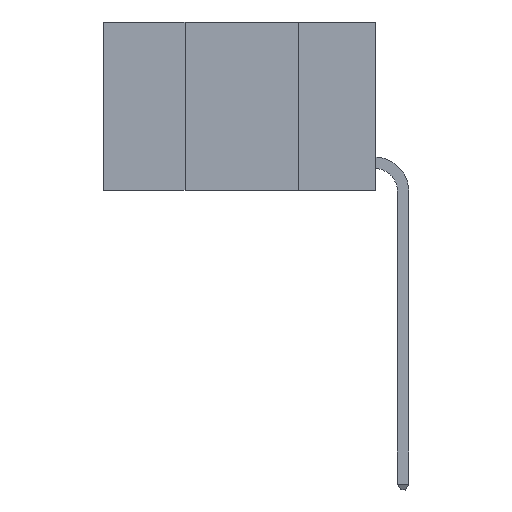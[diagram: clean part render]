
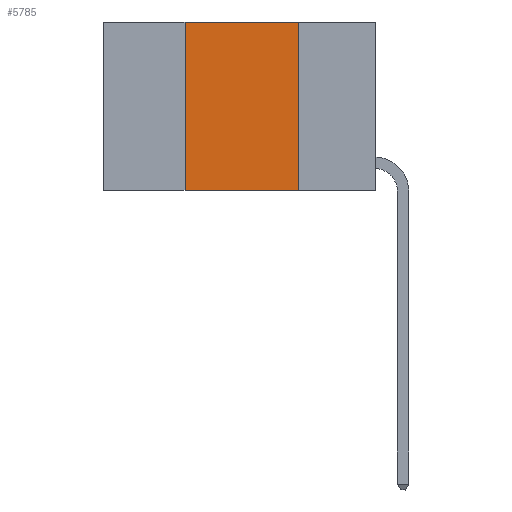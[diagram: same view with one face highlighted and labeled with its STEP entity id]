
A CAD part, left-side view. The second image highlights one B-rep face of the part: STEP entity #5785.
In plain terms, the highlighted planar face has unit normal (-1, 0, 0).
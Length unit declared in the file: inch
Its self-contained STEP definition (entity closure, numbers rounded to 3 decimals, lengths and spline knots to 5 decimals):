
#475 = LINE ( 'NONE', #14678, #10273 ) ;
#1398 = VERTEX_POINT ( 'NONE', #12141 ) ;
#1411 = LINE ( 'NONE', #5792, #14054 ) ;
#2137 = DIRECTION ( 'NONE',  ( 0., -1., 0. ) ) ;
#2446 = ORIENTED_EDGE ( 'NONE', *, *, #2503, .F. ) ;
#2503 = EDGE_CURVE ( 'NONE', #8570, #13165, #1411, .T. ) ;
#3089 = ORIENTED_EDGE ( 'NONE', *, *, #15133, .T. ) ;
#3244 = CARTESIAN_POINT ( 'NONE',  ( 0., 0.17, -0.37 ) ) ;
#3879 = FACE_OUTER_BOUND ( 'NONE', #5283, .T. ) ;
#4567 = DIRECTION ( 'NONE',  ( 1., 0., 0. ) ) ;
#5283 = EDGE_LOOP ( 'NONE', ( #5340, #2446, #15800, #3089 ) ) ;
#5340 = ORIENTED_EDGE ( 'NONE', *, *, #11957, .F. ) ;
#5511 = CARTESIAN_POINT ( 'NONE',  ( 0., 0.42, 0. ) ) ;
#5785 = ADVANCED_FACE ( 'NONE', ( #3879 ), #8215, .F. ) ;
#5792 = CARTESIAN_POINT ( 'NONE',  ( 0., 0.6, 0. ) ) ;
#6228 = CARTESIAN_POINT ( 'NONE',  ( 0., 0.17, 0. ) ) ;
#6819 = AXIS2_PLACEMENT_3D ( 'NONE', #8270, #4567, #13163 ) ;
#7413 = DIRECTION ( 'NONE',  ( 0., -1., 0. ) ) ;
#7443 = LINE ( 'NONE', #5511, #10307 ) ;
#8056 = VECTOR ( 'NONE', #8723, 39.37008 ) ;
#8215 = PLANE ( 'NONE',  #6819 ) ;
#8270 = CARTESIAN_POINT ( 'NONE',  ( 0., 0.6, 0. ) ) ;
#8570 = VERTEX_POINT ( 'NONE', #15710 ) ;
#8723 = DIRECTION ( 'NONE',  ( 0., 0., -1. ) ) ;
#10273 = VECTOR ( 'NONE', #7413, 39.37008 ) ;
#10307 = VECTOR ( 'NONE', #15275, 39.37008 ) ;
#11287 = LINE ( 'NONE', #6228, #8056 ) ;
#11957 = EDGE_CURVE ( 'NONE', #13165, #14898, #11287, .T. ) ;
#12141 = CARTESIAN_POINT ( 'NONE',  ( 0., 0.42, -0.37 ) ) ;
#13163 = DIRECTION ( 'NONE',  ( 0., 0., -1. ) ) ;
#13165 = VERTEX_POINT ( 'NONE', #14514 ) ;
#14054 = VECTOR ( 'NONE', #2137, 39.37008 ) ;
#14275 = EDGE_CURVE ( 'NONE', #1398, #8570, #7443, .T. ) ;
#14514 = CARTESIAN_POINT ( 'NONE',  ( 0., 0.17, 0. ) ) ;
#14678 = CARTESIAN_POINT ( 'NONE',  ( 0., 0.6, -0.37 ) ) ;
#14898 = VERTEX_POINT ( 'NONE', #3244 ) ;
#15133 = EDGE_CURVE ( 'NONE', #1398, #14898, #475, .T. ) ;
#15275 = DIRECTION ( 'NONE',  ( 0., 0., 1. ) ) ;
#15710 = CARTESIAN_POINT ( 'NONE',  ( 0., 0.42, 0. ) ) ;
#15800 = ORIENTED_EDGE ( 'NONE', *, *, #14275, .F. ) ;
